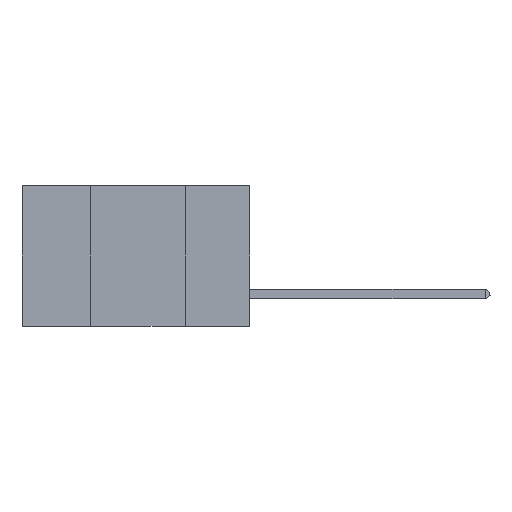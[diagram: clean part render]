
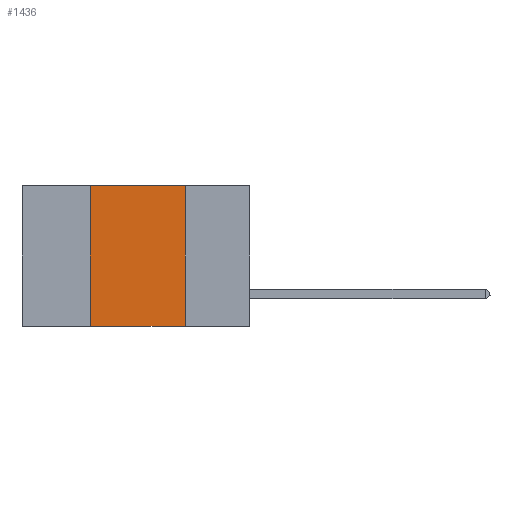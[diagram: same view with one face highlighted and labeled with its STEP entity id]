
A CAD part, left-side view. The second image highlights one B-rep face of the part: STEP entity #1436.
In plain terms, the highlighted planar face has unit normal (-1, 0, 0).
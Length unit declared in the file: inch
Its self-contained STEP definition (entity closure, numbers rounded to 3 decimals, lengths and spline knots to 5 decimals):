
#187 = VERTEX_POINT ( 'NONE', #12078 ) ;
#946 = LINE ( 'NONE', #17275, #1604 ) ;
#1436 = ADVANCED_FACE ( 'NONE', ( #6635 ), #3768, .F. ) ;
#1505 = VECTOR ( 'NONE', #4662, 39.37008 ) ;
#1604 = VECTOR ( 'NONE', #14531, 39.37008 ) ;
#3299 = CARTESIAN_POINT ( 'NONE',  ( 0., 0.6, 0. ) ) ;
#3768 = PLANE ( 'NONE',  #7601 ) ;
#3905 = VECTOR ( 'NONE', #13614, 39.37008 ) ;
#4662 = DIRECTION ( 'NONE',  ( 0., -1., 0. ) ) ;
#4728 = DIRECTION ( 'NONE',  ( 0., 0., 1. ) ) ;
#5342 = LINE ( 'NONE', #11673, #10835 ) ;
#6635 = FACE_OUTER_BOUND ( 'NONE', #16211, .T. ) ;
#6682 = DIRECTION ( 'NONE',  ( 1., 0., 0. ) ) ;
#6759 = ORIENTED_EDGE ( 'NONE', *, *, #13338, .F. ) ;
#6802 = VERTEX_POINT ( 'NONE', #15744 ) ;
#7338 = ORIENTED_EDGE ( 'NONE', *, *, #7831, .T. ) ;
#7601 = AXIS2_PLACEMENT_3D ( 'NONE', #11957, #6682, #13381 ) ;
#7831 = EDGE_CURVE ( 'NONE', #6802, #11996, #946, .T. ) ;
#7861 = CARTESIAN_POINT ( 'NONE',  ( 0., 0.17, -0.37 ) ) ;
#8008 = CARTESIAN_POINT ( 'NONE',  ( 0., 0.42, 0. ) ) ;
#8542 = LINE ( 'NONE', #14943, #3905 ) ;
#10835 = VECTOR ( 'NONE', #4728, 39.37008 ) ;
#11006 = EDGE_CURVE ( 'NONE', #6802, #15752, #5342, .T. ) ;
#11673 = CARTESIAN_POINT ( 'NONE',  ( 0., 0.42, 0. ) ) ;
#11957 = CARTESIAN_POINT ( 'NONE',  ( 0., 0.6, 0. ) ) ;
#11996 = VERTEX_POINT ( 'NONE', #7861 ) ;
#12078 = CARTESIAN_POINT ( 'NONE',  ( 0., 0.17, 0. ) ) ;
#13338 = EDGE_CURVE ( 'NONE', #187, #11996, #8542, .T. ) ;
#13381 = DIRECTION ( 'NONE',  ( 0., 0., -1. ) ) ;
#13577 = LINE ( 'NONE', #3299, #1505 ) ;
#13614 = DIRECTION ( 'NONE',  ( 0., 0., -1. ) ) ;
#14078 = EDGE_CURVE ( 'NONE', #15752, #187, #13577, .T. ) ;
#14531 = DIRECTION ( 'NONE',  ( 0., -1., 0. ) ) ;
#14560 = ORIENTED_EDGE ( 'NONE', *, *, #14078, .F. ) ;
#14943 = CARTESIAN_POINT ( 'NONE',  ( 0., 0.17, 0. ) ) ;
#15012 = ORIENTED_EDGE ( 'NONE', *, *, #11006, .F. ) ;
#15744 = CARTESIAN_POINT ( 'NONE',  ( 0., 0.42, -0.37 ) ) ;
#15752 = VERTEX_POINT ( 'NONE', #8008 ) ;
#16211 = EDGE_LOOP ( 'NONE', ( #6759, #14560, #15012, #7338 ) ) ;
#17275 = CARTESIAN_POINT ( 'NONE',  ( 0., 0.6, -0.37 ) ) ;
